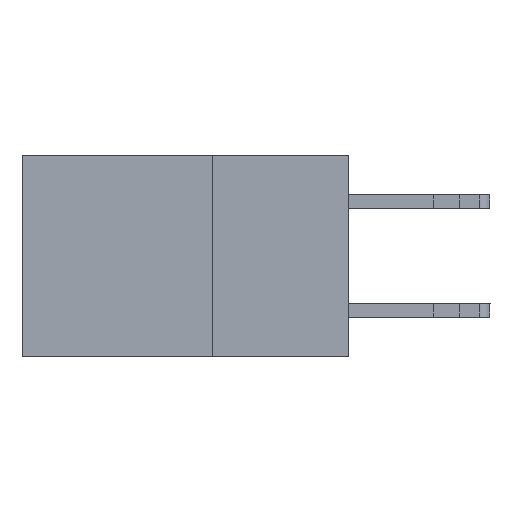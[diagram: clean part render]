
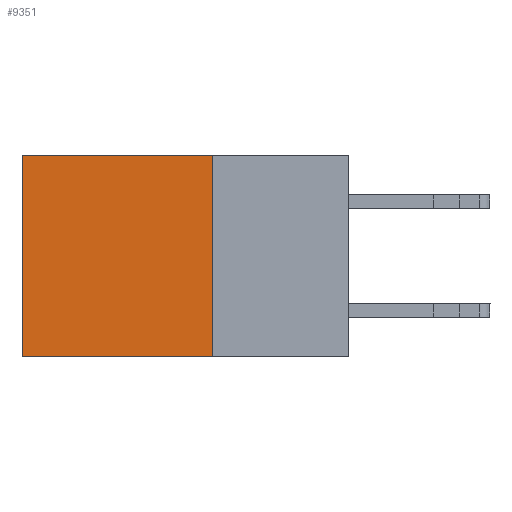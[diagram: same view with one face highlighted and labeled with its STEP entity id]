
A CAD part, left-side view. The second image highlights one B-rep face of the part: STEP entity #9351.
In plain terms, the highlighted planar face has unit normal (-1, 0, 0).
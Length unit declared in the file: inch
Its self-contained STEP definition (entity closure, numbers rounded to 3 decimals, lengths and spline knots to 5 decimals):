
#825 = VECTOR ( 'NONE', #12530, 39.37008 ) ;
#1116 = VERTEX_POINT ( 'NONE', #2934 ) ;
#1244 = VERTEX_POINT ( 'NONE', #10879 ) ;
#1514 = LINE ( 'NONE', #6211, #3642 ) ;
#1527 = EDGE_CURVE ( 'NONE', #1116, #1244, #12722, .T. ) ;
#2934 = CARTESIAN_POINT ( 'NONE',  ( 0.298, 0.25, 0. ) ) ;
#3100 = EDGE_CURVE ( 'NONE', #3980, #6503, #10104, .T. ) ;
#3288 = CARTESIAN_POINT ( 'NONE',  ( 0.298, 0.6, -0.37 ) ) ;
#3642 = VECTOR ( 'NONE', #4987, 39.37008 ) ;
#3771 = CARTESIAN_POINT ( 'NONE',  ( 0.298, 0.6, 0. ) ) ;
#3809 = DIRECTION ( 'NONE',  ( 1., 0., 0. ) ) ;
#3858 = CARTESIAN_POINT ( 'NONE',  ( 0.298, 0.25, 0. ) ) ;
#3958 = ORIENTED_EDGE ( 'NONE', *, *, #1527, .T. ) ;
#3980 = VERTEX_POINT ( 'NONE', #9724 ) ;
#4987 = DIRECTION ( 'NONE',  ( 0., 0., -1. ) ) ;
#5794 = ORIENTED_EDGE ( 'NONE', *, *, #3100, .F. ) ;
#5829 = LINE ( 'NONE', #3771, #6167 ) ;
#6167 = VECTOR ( 'NONE', #10743, 39.37008 ) ;
#6211 = CARTESIAN_POINT ( 'NONE',  ( 0.298, 0.25, 0. ) ) ;
#6503 = VERTEX_POINT ( 'NONE', #3288 ) ;
#8522 = CARTESIAN_POINT ( 'NONE',  ( 0.298, 0.25, 0. ) ) ;
#8648 = EDGE_CURVE ( 'NONE', #1116, #3980, #1514, .T. ) ;
#9351 = ADVANCED_FACE ( 'NONE', ( #13688 ), #10555, .F. ) ;
#9484 = ORIENTED_EDGE ( 'NONE', *, *, #11540, .T. ) ;
#9705 = DIRECTION ( 'NONE',  ( 0., 1., 0. ) ) ;
#9724 = CARTESIAN_POINT ( 'NONE',  ( 0.298, 0.25, -0.37 ) ) ;
#9851 = ORIENTED_EDGE ( 'NONE', *, *, #8648, .F. ) ;
#10104 = LINE ( 'NONE', #11529, #825 ) ;
#10555 = PLANE ( 'NONE',  #10963 ) ;
#10743 = DIRECTION ( 'NONE',  ( 0., 0., -1. ) ) ;
#10879 = CARTESIAN_POINT ( 'NONE',  ( 0.298, 0.6, 0. ) ) ;
#10963 = AXIS2_PLACEMENT_3D ( 'NONE', #3858, #3809, #11654 ) ;
#11011 = VECTOR ( 'NONE', #9705, 39.37008 ) ;
#11426 = EDGE_LOOP ( 'NONE', ( #9484, #5794, #9851, #3958 ) ) ;
#11529 = CARTESIAN_POINT ( 'NONE',  ( 0.298, 0.25, -0.37 ) ) ;
#11540 = EDGE_CURVE ( 'NONE', #1244, #6503, #5829, .T. ) ;
#11654 = DIRECTION ( 'NONE',  ( 0., 0., -1. ) ) ;
#12530 = DIRECTION ( 'NONE',  ( 0., 1., 0. ) ) ;
#12722 = LINE ( 'NONE', #8522, #11011 ) ;
#13688 = FACE_OUTER_BOUND ( 'NONE', #11426, .T. ) ;
